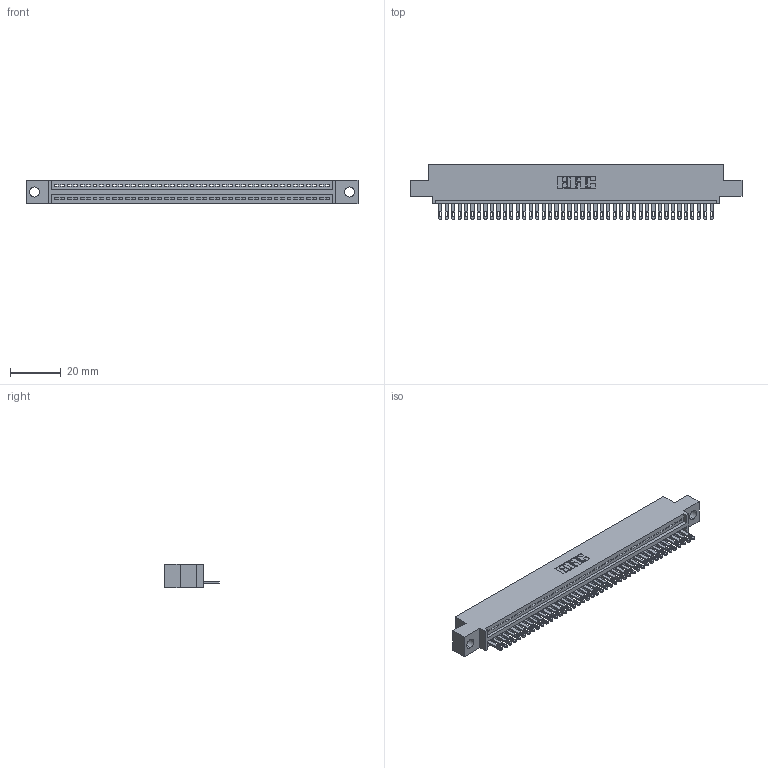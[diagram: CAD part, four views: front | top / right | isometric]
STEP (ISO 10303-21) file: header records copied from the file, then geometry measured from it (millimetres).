
FILE_DESCRIPTION (( 'STEP AP203' ), '1' );
FILE_NAME ('345-043-500-404.STEP', '2021-05-26T15:03:33', ( '' ), ( '' ), 'SwSTEP 2.0', 'SolidWorks 2020', '' );
FILE_SCHEMA (( 'CONFIG_CONTROL_DESIGN' ));
Length unit declared in the file: inch
Products named in the file (3): 345 Part_0.110 Offset - 0.156 Dia-TI; 345-043-500-404; 345-292-001_345-293-100
Assembly tree (44 placements, depth 2):
  345-043-500-404
    345 Part_0.110 Offset - 0.156 Dia-TI
    345-292-001_345-293-100  x43
Bounding box: 130.43 x 21.51 x 9.4 mm (x, y, z)
Volume: 12243.8 mm3; surface area: 16305.4 mm2
Topology: 44 solids, 44 shells, 2466 faces, 7613 edges, 5074 vertices
Faces by surface type: plane 1560, cylinder 906
Entity records: 32709 total; most frequent: CARTESIAN_POINT 5675, ORIENTED_EDGE 5650, DIRECTION 4955, EDGE_CURVE 2825, VECTOR 2517, LINE 2517, VERTEX_POINT 1882, AXIS2_PLACEMENT_3D 1219
